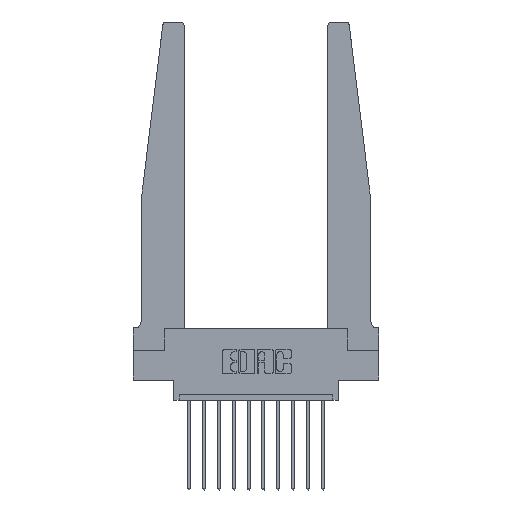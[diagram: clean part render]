
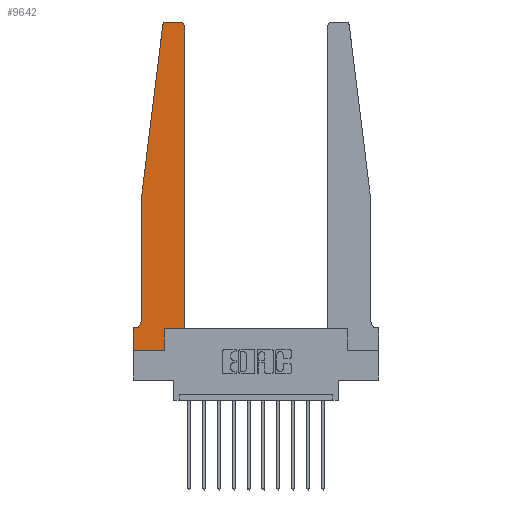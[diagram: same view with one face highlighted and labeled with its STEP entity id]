
A CAD part, top view. The second image highlights one B-rep face of the part: STEP entity #9642.
In plain terms, the highlighted planar face has unit normal (0, 0, 1).
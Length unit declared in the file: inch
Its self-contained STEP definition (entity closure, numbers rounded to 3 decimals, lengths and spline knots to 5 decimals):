
#107 = CARTESIAN_POINT ( 'NONE',  ( 0.27653, 2.75, 0.37 ) ) ;
#155 = CARTESIAN_POINT ( 'NONE',  ( 0.27653, 2.72, 0.37 ) ) ;
#529 = DIRECTION ( 'NONE',  ( -1., 0., 0. ) ) ;
#578 = AXIS2_PLACEMENT_3D ( 'NONE', #2676, #11848, #15327 ) ;
#685 = VERTEX_POINT ( 'NONE', #1277 ) ;
#1088 = DIRECTION ( 'NONE',  ( -1., 0., 0. ) ) ;
#1277 = CARTESIAN_POINT ( 'NONE',  ( 0.2605, 0., 0.37 ) ) ;
#1454 = VECTOR ( 'NONE', #8783, 39.37008 ) ;
#1777 = LINE ( 'NONE', #13392, #1974 ) ;
#1808 = CARTESIAN_POINT ( 'NONE',  ( 0.065, 0.1875, 0.37 ) ) ;
#1933 = ORIENTED_EDGE ( 'NONE', *, *, #4166, .T. ) ;
#1941 = DIRECTION ( 'NONE',  ( -0.122, -0.992, 0. ) ) ;
#1967 = VERTEX_POINT ( 'NONE', #107 ) ;
#1974 = VECTOR ( 'NONE', #2598, 39.37008 ) ;
#2150 = CIRCLE ( 'NONE', #13301, 0.05 ) ;
#2211 = AXIS2_PLACEMENT_3D ( 'NONE', #2476, #9604, #9449 ) ;
#2275 = CARTESIAN_POINT ( 'NONE',  ( 0.2605, 0.18, 0.37 ) ) ;
#2476 = CARTESIAN_POINT ( 'NONE',  ( 0.395, 2.72, 0.37 ) ) ;
#2598 = DIRECTION ( 'NONE',  ( 0., 1., 0. ) ) ;
#2676 = CARTESIAN_POINT ( 'NONE',  ( 0., 0.1875, 0.37 ) ) ;
#2703 = VECTOR ( 'NONE', #1088, 39.37008 ) ;
#2833 = CARTESIAN_POINT ( 'NONE',  ( 0.015, 0.2375, 0.37 ) ) ;
#2912 = EDGE_CURVE ( 'NONE', #9478, #14756, #13561, .T. ) ;
#2923 = CARTESIAN_POINT ( 'NONE',  ( 0.065, 0.2375, 0.37 ) ) ;
#3195 = EDGE_CURVE ( 'NONE', #11364, #4410, #2150, .T. ) ;
#3438 = CARTESIAN_POINT ( 'NONE',  ( 0.425, 0.18, 0.37 ) ) ;
#3640 = LINE ( 'NONE', #12951, #6618 ) ;
#3727 = DIRECTION ( 'NONE',  ( 1., 0., 0. ) ) ;
#4166 = EDGE_CURVE ( 'NONE', #12356, #685, #7331, .T. ) ;
#4410 = VERTEX_POINT ( 'NONE', #9759 ) ;
#4426 = EDGE_CURVE ( 'NONE', #13831, #11364, #9803, .T. ) ;
#4720 = VERTEX_POINT ( 'NONE', #2275 ) ;
#4782 = DIRECTION ( 'NONE',  ( 0., 0., 1. ) ) ;
#4867 = EDGE_CURVE ( 'NONE', #1967, #13620, #13493, .T. ) ;
#4899 = CARTESIAN_POINT ( 'NONE',  ( 0.065, 1.25, 0.37 ) ) ;
#5044 = LINE ( 'NONE', #11388, #12175 ) ;
#5293 = VECTOR ( 'NONE', #13813, 39.37008 ) ;
#5551 = CARTESIAN_POINT ( 'NONE',  ( 0., 0., 0.37 ) ) ;
#5725 = AXIS2_PLACEMENT_3D ( 'NONE', #155, #4782, #3727 ) ;
#6368 = ORIENTED_EDGE ( 'NONE', *, *, #13606, .T. ) ;
#6618 = VECTOR ( 'NONE', #9333, 39.37008 ) ;
#6636 = ORIENTED_EDGE ( 'NONE', *, *, #11928, .T. ) ;
#6777 = ORIENTED_EDGE ( 'NONE', *, *, #9213, .T. ) ;
#6890 = CARTESIAN_POINT ( 'NONE',  ( 0.24675, 2.72367, 0.37 ) ) ;
#7158 = PLANE ( 'NONE',  #578 ) ;
#7331 = LINE ( 'NONE', #5551, #5293 ) ;
#7538 = VECTOR ( 'NONE', #13376, 39.37008 ) ;
#7715 = CARTESIAN_POINT ( 'NONE',  ( 0.425, 2.72, 0.37 ) ) ;
#7824 = ORIENTED_EDGE ( 'NONE', *, *, #2912, .T. ) ;
#8783 = DIRECTION ( 'NONE',  ( 0., 1., 0. ) ) ;
#8845 = ORIENTED_EDGE ( 'NONE', *, *, #12996, .T. ) ;
#8856 = DIRECTION ( 'NONE',  ( -1., 0., 0. ) ) ;
#9139 = CARTESIAN_POINT ( 'NONE',  ( 0.395, 2.75, 0.37 ) ) ;
#9171 = FACE_OUTER_BOUND ( 'NONE', #12983, .T. ) ;
#9213 = EDGE_CURVE ( 'NONE', #9914, #12356, #12170, .T. ) ;
#9333 = DIRECTION ( 'NONE',  ( 1., 0., 0. ) ) ;
#9368 = ORIENTED_EDGE ( 'NONE', *, *, #4426, .T. ) ;
#9449 = DIRECTION ( 'NONE',  ( 1., 0., 0. ) ) ;
#9478 = VERTEX_POINT ( 'NONE', #7715 ) ;
#9604 = DIRECTION ( 'NONE',  ( 0., 0., 1. ) ) ;
#9642 = ADVANCED_FACE ( 'NONE', ( #9171 ), #7158, .T. ) ;
#9759 = CARTESIAN_POINT ( 'NONE',  ( 0.015, 0.1875, 0.37 ) ) ;
#9803 = LINE ( 'NONE', #13422, #7538 ) ;
#9883 = VECTOR ( 'NONE', #529, 39.37008 ) ;
#9914 = VERTEX_POINT ( 'NONE', #10078 ) ;
#10015 = EDGE_CURVE ( 'NONE', #13620, #13831, #5044, .T. ) ;
#10078 = CARTESIAN_POINT ( 'NONE',  ( 0., 0.1875, 0.37 ) ) ;
#10172 = DIRECTION ( 'NONE',  ( 0., 0., -1. ) ) ;
#10605 = CARTESIAN_POINT ( 'NONE',  ( 0.25, 2.75, 0.37 ) ) ;
#11200 = LINE ( 'NONE', #1808, #9883 ) ;
#11364 = VERTEX_POINT ( 'NONE', #2923 ) ;
#11388 = CARTESIAN_POINT ( 'NONE',  ( 0.065, 1.25, 0.37 ) ) ;
#11400 = EDGE_CURVE ( 'NONE', #685, #4720, #14161, .T. ) ;
#11533 = LINE ( 'NONE', #10605, #2703 ) ;
#11775 = CARTESIAN_POINT ( 'NONE',  ( 0., 0., 0.37 ) ) ;
#11811 = VECTOR ( 'NONE', #12252, 39.37008 ) ;
#11848 = DIRECTION ( 'NONE',  ( 0., 0., 1. ) ) ;
#11928 = EDGE_CURVE ( 'NONE', #4410, #9914, #11200, .T. ) ;
#12170 = LINE ( 'NONE', #14574, #11811 ) ;
#12175 = VECTOR ( 'NONE', #1941, 39.37008 ) ;
#12252 = DIRECTION ( 'NONE',  ( 0., -1., 0. ) ) ;
#12311 = ORIENTED_EDGE ( 'NONE', *, *, #4867, .T. ) ;
#12335 = VERTEX_POINT ( 'NONE', #3438 ) ;
#12356 = VERTEX_POINT ( 'NONE', #11775 ) ;
#12951 = CARTESIAN_POINT ( 'NONE',  ( 0.425, 0.18, 0.37 ) ) ;
#12983 = EDGE_LOOP ( 'NONE', ( #6368, #12311, #13729, #9368, #14879, #6636, #6777, #1933, #14290, #14282, #8845, #7824 ) ) ;
#12996 = EDGE_CURVE ( 'NONE', #12335, #9478, #1777, .T. ) ;
#13301 = AXIS2_PLACEMENT_3D ( 'NONE', #2833, #10172, #8856 ) ;
#13376 = DIRECTION ( 'NONE',  ( 0., -1., 0. ) ) ;
#13392 = CARTESIAN_POINT ( 'NONE',  ( 0.425, 0.18, 0.37 ) ) ;
#13422 = CARTESIAN_POINT ( 'NONE',  ( 0.065, 1.25, 0.37 ) ) ;
#13493 = CIRCLE ( 'NONE', #5725, 0.03 ) ;
#13561 = CIRCLE ( 'NONE', #2211, 0.03 ) ;
#13606 = EDGE_CURVE ( 'NONE', #14756, #1967, #11533, .T. ) ;
#13620 = VERTEX_POINT ( 'NONE', #6890 ) ;
#13667 = EDGE_CURVE ( 'NONE', #4720, #12335, #3640, .T. ) ;
#13669 = CARTESIAN_POINT ( 'NONE',  ( 0.2605, 0.18, 0.37 ) ) ;
#13729 = ORIENTED_EDGE ( 'NONE', *, *, #10015, .T. ) ;
#13813 = DIRECTION ( 'NONE',  ( 1., 0., 0. ) ) ;
#13831 = VERTEX_POINT ( 'NONE', #4899 ) ;
#14161 = LINE ( 'NONE', #13669, #1454 ) ;
#14282 = ORIENTED_EDGE ( 'NONE', *, *, #13667, .T. ) ;
#14290 = ORIENTED_EDGE ( 'NONE', *, *, #11400, .T. ) ;
#14574 = CARTESIAN_POINT ( 'NONE',  ( 0., 0., 0.37 ) ) ;
#14756 = VERTEX_POINT ( 'NONE', #9139 ) ;
#14879 = ORIENTED_EDGE ( 'NONE', *, *, #3195, .T. ) ;
#15327 = DIRECTION ( 'NONE',  ( 1., 0., 0. ) ) ;
